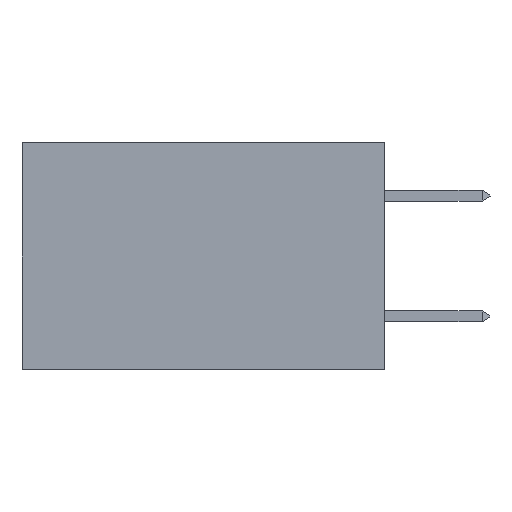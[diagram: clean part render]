
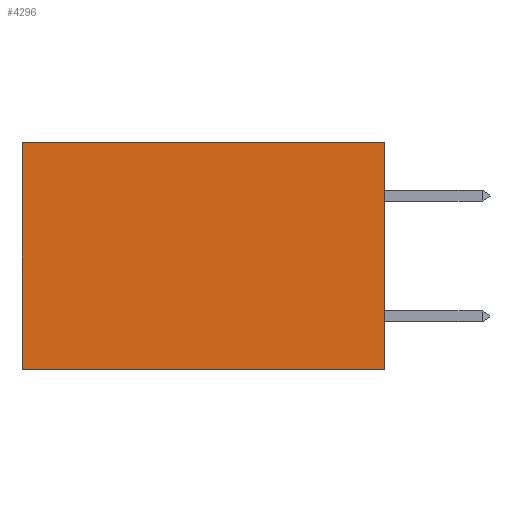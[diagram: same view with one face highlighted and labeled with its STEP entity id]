
A CAD part, left-side view. The second image highlights one B-rep face of the part: STEP entity #4296.
In plain terms, the highlighted planar face has unit normal (-1, 0, 0).
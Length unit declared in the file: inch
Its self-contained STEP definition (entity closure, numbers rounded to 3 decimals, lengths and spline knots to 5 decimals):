
#67 = CARTESIAN_POINT ( 'NONE',  ( 0.2875, 0.6, -0.375 ) ) ;
#572 = VECTOR ( 'NONE', #12579, 39.37008 ) ;
#613 = DIRECTION ( 'NONE',  ( 0., 0., -1. ) ) ;
#816 = FACE_OUTER_BOUND ( 'NONE', #6264, .T. ) ;
#1396 = AXIS2_PLACEMENT_3D ( 'NONE', #5740, #11965, #613 ) ;
#1717 = CARTESIAN_POINT ( 'NONE',  ( 0.2875, 0.6, -0.375 ) ) ;
#1891 = VECTOR ( 'NONE', #4658, 39.37008 ) ;
#2476 = VERTEX_POINT ( 'NONE', #9721 ) ;
#3511 = DIRECTION ( 'NONE',  ( 0., 1., 0. ) ) ;
#3999 = ORIENTED_EDGE ( 'NONE', *, *, #8574, .T. ) ;
#4131 = ORIENTED_EDGE ( 'NONE', *, *, #5578, .F. ) ;
#4296 = ADVANCED_FACE ( 'NONE', ( #816 ), #6897, .F. ) ;
#4331 = CARTESIAN_POINT ( 'NONE',  ( 0.2875, 0., 0. ) ) ;
#4398 = ORIENTED_EDGE ( 'NONE', *, *, #7855, .F. ) ;
#4477 = VERTEX_POINT ( 'NONE', #8196 ) ;
#4658 = DIRECTION ( 'NONE',  ( 0., 1., 0. ) ) ;
#4721 = CARTESIAN_POINT ( 'NONE',  ( 0.2875, 0., -0.375 ) ) ;
#4724 = DIRECTION ( 'NONE',  ( 0., 0., -1. ) ) ;
#4862 = LINE ( 'NONE', #4721, #1891 ) ;
#5578 = EDGE_CURVE ( 'NONE', #2476, #4477, #7995, .T. ) ;
#5740 = CARTESIAN_POINT ( 'NONE',  ( 0.2875, 0., -0.375 ) ) ;
#5936 = CARTESIAN_POINT ( 'NONE',  ( 0.2875, 0.6, 0. ) ) ;
#6264 = EDGE_LOOP ( 'NONE', ( #11778, #4398, #4131, #3999 ) ) ;
#6382 = LINE ( 'NONE', #4331, #11506 ) ;
#6897 = PLANE ( 'NONE',  #1396 ) ;
#7855 = EDGE_CURVE ( 'NONE', #4477, #12772, #4862, .T. ) ;
#7995 = LINE ( 'NONE', #11153, #9746 ) ;
#8196 = CARTESIAN_POINT ( 'NONE',  ( 0.2875, 0., -0.375 ) ) ;
#8574 = EDGE_CURVE ( 'NONE', #2476, #13464, #6382, .T. ) ;
#8973 = EDGE_CURVE ( 'NONE', #13464, #12772, #12452, .T. ) ;
#9721 = CARTESIAN_POINT ( 'NONE',  ( 0.2875, 0., 0. ) ) ;
#9746 = VECTOR ( 'NONE', #4724, 39.37008 ) ;
#11153 = CARTESIAN_POINT ( 'NONE',  ( 0.2875, 0., -0.375 ) ) ;
#11506 = VECTOR ( 'NONE', #3511, 39.37008 ) ;
#11778 = ORIENTED_EDGE ( 'NONE', *, *, #8973, .T. ) ;
#11965 = DIRECTION ( 'NONE',  ( 1., 0., 0. ) ) ;
#12452 = LINE ( 'NONE', #67, #572 ) ;
#12579 = DIRECTION ( 'NONE',  ( 0., 0., -1. ) ) ;
#12772 = VERTEX_POINT ( 'NONE', #1717 ) ;
#13464 = VERTEX_POINT ( 'NONE', #5936 ) ;
